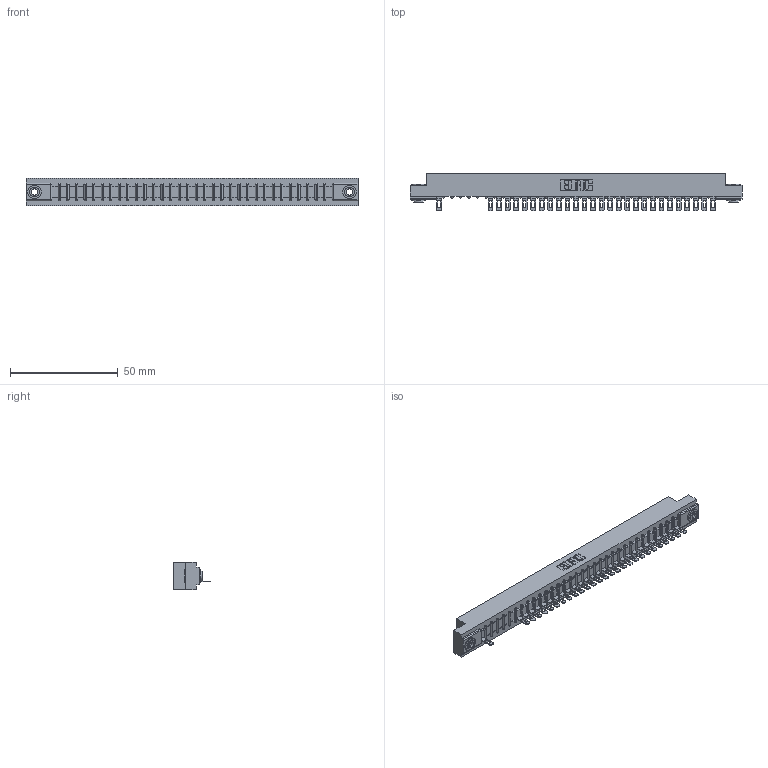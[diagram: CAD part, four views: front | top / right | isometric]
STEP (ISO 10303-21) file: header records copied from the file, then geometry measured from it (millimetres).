
FILE_DESCRIPTION (( 'STEP AP203' ), '1' );
FILE_NAME ('357-033-501-103.STEP', '2018-08-10T01:19:34', ( '' ), ( '' ), 'SwSTEP 2.0', 'SolidWorks 2016', '' );
FILE_SCHEMA (( 'CONFIG_CONTROL_DESIGN' ));
Length unit declared in the file: inch
Products named in the file (4): 307 Part_.156 Dia Mounting Holes; 307-290-002_501; 345-250-002_345-250-002-102; 357-033-501-103
Assembly tree (31 placements, depth 2):
  357-033-501-103
    307 Part_.156 Dia Mounting Holes
    307-290-002_501  x28
    345-250-002_345-250-002-102  x2
Bounding box: 153.77 x 17.42 x 12.7 mm (x, y, z)
Volume: 16269.4 mm3; surface area: 19771.1 mm2
Topology: 31 solids, 31 shells, 2432 faces, 7419 edges, 4850 vertices
Faces by surface type: plane 1386, cylinder 970, sphere 68, cone 8
Entity records: 31099 total; most frequent: CARTESIAN_POINT 5244, ORIENTED_EDGE 5230, DIRECTION 5113, EDGE_CURVE 2615, VECTOR 1987, LINE 1987, VERTEX_POINT 1694, AXIS2_PLACEMENT_3D 1563
